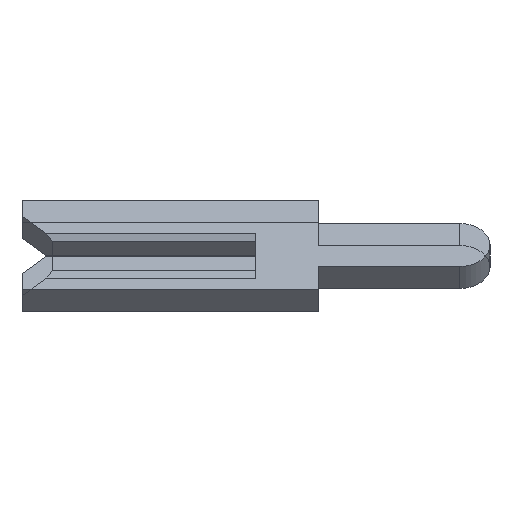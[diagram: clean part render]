
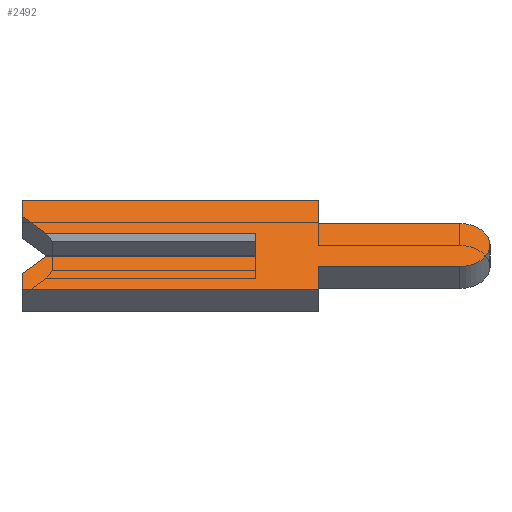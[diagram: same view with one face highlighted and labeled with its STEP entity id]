
A CAD part, left-side view. The second image highlights one B-rep face of the part: STEP entity #2492.
In plain terms, the highlighted face is planar.
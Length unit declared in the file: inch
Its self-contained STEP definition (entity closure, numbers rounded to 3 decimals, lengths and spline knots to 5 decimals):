
#36 = CARTESIAN_POINT ( 'NONE',  ( -0.01, 0.15, -0.04 ) ) ;
#107 = EDGE_CURVE ( 'NONE', #3180, #2590, #1143, .T. ) ;
#114 = CARTESIAN_POINT ( 'NONE',  ( -0.01, -0.04, 0.04 ) ) ;
#148 = VECTOR ( 'NONE', #1186, 39.37008 ) ;
#223 = ORIENTED_EDGE ( 'NONE', *, *, #336, .F. ) ;
#240 = ORIENTED_EDGE ( 'NONE', *, *, #3770, .F. ) ;
#252 = CARTESIAN_POINT ( 'NONE',  ( -0.01, 0.134, 0.01 ) ) ;
#256 = LINE ( 'NONE', #728, #2222 ) ;
#263 = VERTEX_POINT ( 'NONE', #923 ) ;
#294 = CARTESIAN_POINT ( 'NONE',  ( -0.01, -0.1305, 0.0195 ) ) ;
#305 = VECTOR ( 'NONE', #3773, 39.37008 ) ;
#336 = EDGE_CURVE ( 'NONE', #2750, #3180, #2020, .T. ) ;
#363 = DIRECTION ( 'NONE',  ( 0., -1., 0. ) ) ;
#417 = LINE ( 'NONE', #1323, #3799 ) ;
#418 = CARTESIAN_POINT ( 'NONE',  ( -0.01, 0., -0.01 ) ) ;
#441 = LINE ( 'NONE', #848, #148 ) ;
#448 = CARTESIAN_POINT ( 'NONE',  ( -0.01, -0.04, -0.0195 ) ) ;
#514 = CARTESIAN_POINT ( 'NONE',  ( -0.01, 0.15, -0.026 ) ) ;
#549 = LINE ( 'NONE', #2681, #627 ) ;
#596 = CARTESIAN_POINT ( 'NONE',  ( -0.01, -0.1305, 0. ) ) ;
#627 = VECTOR ( 'NONE', #901, 39.37008 ) ;
#654 = DIRECTION ( 'NONE',  ( 0., 1., 0. ) ) ;
#665 = LINE ( 'NONE', #2844, #951 ) ;
#690 = EDGE_CURVE ( 'NONE', #2633, #2304, #3844, .T. ) ;
#728 = CARTESIAN_POINT ( 'NONE',  ( -0.01, 0.15, 0.04 ) ) ;
#785 = CARTESIAN_POINT ( 'NONE',  ( -0.01, 0.15, -0.04 ) ) ;
#789 = ORIENTED_EDGE ( 'NONE', *, *, #107, .F. ) ;
#848 = CARTESIAN_POINT ( 'NONE',  ( -0.01, -0.04, -0.0195 ) ) ;
#854 = CIRCLE ( 'NONE', #2845, 0.0195 ) ;
#872 = EDGE_CURVE ( 'NONE', #2750, #1251, #417, .T. ) ;
#901 = DIRECTION ( 'NONE',  ( 0., -1., 0. ) ) ;
#919 = CARTESIAN_POINT ( 'NONE',  ( -0.01, 0.15, 0.026 ) ) ;
#923 = CARTESIAN_POINT ( 'NONE',  ( -0.01, -0.1305, -0.0195 ) ) ;
#929 = DIRECTION ( 'NONE',  ( 1., 0., 0. ) ) ;
#931 = VECTOR ( 'NONE', #654, 39.37008 ) ;
#951 = VECTOR ( 'NONE', #2807, 39.37008 ) ;
#999 = EDGE_CURVE ( 'NONE', #2590, #2348, #256, .T. ) ;
#1027 = EDGE_CURVE ( 'NONE', #2304, #2015, #2981, .T. ) ;
#1065 = ORIENTED_EDGE ( 'NONE', *, *, #1729, .F. ) ;
#1084 = CARTESIAN_POINT ( 'NONE',  ( -0.01, -0.04, -0.04 ) ) ;
#1143 = LINE ( 'NONE', #2137, #2611 ) ;
#1186 = DIRECTION ( 'NONE',  ( 0., 1., 0. ) ) ;
#1193 = ORIENTED_EDGE ( 'NONE', *, *, #2713, .F. ) ;
#1248 = DIRECTION ( 'NONE',  ( 0., 0.707, 0.707 ) ) ;
#1251 = VERTEX_POINT ( 'NONE', #2852 ) ;
#1310 = VECTOR ( 'NONE', #3634, 39.37008 ) ;
#1323 = CARTESIAN_POINT ( 'NONE',  ( -0.01, 0.15, 0.01 ) ) ;
#1350 = ORIENTED_EDGE ( 'NONE', *, *, #1027, .F. ) ;
#1370 = CARTESIAN_POINT ( 'NONE',  ( -0.01, 0.1305, -0.0065 ) ) ;
#1396 = VERTEX_POINT ( 'NONE', #448 ) ;
#1451 = EDGE_CURVE ( 'NONE', #1396, #2633, #3030, .T. ) ;
#1494 = CARTESIAN_POINT ( 'NONE',  ( -0.01, 0., 0.0065 ) ) ;
#1647 = EDGE_LOOP ( 'NONE', ( #1805, #1193, #2458, #1065, #1350, #3405, #2413, #3379, #3302, #240, #2543, #2516, #789, #223 ) ) ;
#1671 = CARTESIAN_POINT ( 'NONE',  ( -0.01, 0.15, -0.026 ) ) ;
#1729 = EDGE_CURVE ( 'NONE', #2015, #2900, #3544, .T. ) ;
#1781 = CARTESIAN_POINT ( 'NONE',  ( -0.01, -0.04, -0.04 ) ) ;
#1796 = DIRECTION ( 'NONE',  ( 1., 0., 0. ) ) ;
#1805 = ORIENTED_EDGE ( 'NONE', *, *, #872, .T. ) ;
#1866 = CARTESIAN_POINT ( 'NONE',  ( -0.01, -0.1305, 0. ) ) ;
#2015 = VERTEX_POINT ( 'NONE', #514 ) ;
#2020 = LINE ( 'NONE', #3032, #3547 ) ;
#2052 = PLANE ( 'NONE',  #3288 ) ;
#2083 = DIRECTION ( 'NONE',  ( 0., 0., -1. ) ) ;
#2137 = CARTESIAN_POINT ( 'NONE',  ( -0.01, 0.15, 0.026 ) ) ;
#2222 = VECTOR ( 'NONE', #3177, 39.37008 ) ;
#2225 = VECTOR ( 'NONE', #2865, 39.37008 ) ;
#2304 = VERTEX_POINT ( 'NONE', #785 ) ;
#2335 = CARTESIAN_POINT ( 'NONE',  ( -0.01, -0.04, 0.04 ) ) ;
#2348 = VERTEX_POINT ( 'NONE', #2335 ) ;
#2396 = LINE ( 'NONE', #1494, #1310 ) ;
#2413 = ORIENTED_EDGE ( 'NONE', *, *, #1451, .F. ) ;
#2442 = VERTEX_POINT ( 'NONE', #294 ) ;
#2458 = ORIENTED_EDGE ( 'NONE', *, *, #2512, .F. ) ;
#2467 = DIRECTION ( 'NONE',  ( 0., 0., 1. ) ) ;
#2492 = ADVANCED_FACE ( 'NONE', ( #3735 ), #2052, .F. ) ;
#2506 = DIRECTION ( 'NONE',  ( 0., 0., -1. ) ) ;
#2512 = EDGE_CURVE ( 'NONE', #2900, #3431, #549, .T. ) ;
#2516 = ORIENTED_EDGE ( 'NONE', *, *, #999, .F. ) ;
#2543 = ORIENTED_EDGE ( 'NONE', *, *, #3517, .F. ) ;
#2590 = VERTEX_POINT ( 'NONE', #3339 ) ;
#2611 = VECTOR ( 'NONE', #2467, 39.37008 ) ;
#2633 = VERTEX_POINT ( 'NONE', #1781 ) ;
#2681 = CARTESIAN_POINT ( 'NONE',  ( -0.01, -0.1305, -0.01 ) ) ;
#2713 = EDGE_CURVE ( 'NONE', #3431, #1251, #2396, .T. ) ;
#2717 = CARTESIAN_POINT ( 'NONE',  ( -0.01, -0.04, 0.0195 ) ) ;
#2719 = VECTOR ( 'NONE', #3262, 39.37008 ) ;
#2739 = EDGE_CURVE ( 'NONE', #263, #1396, #441, .T. ) ;
#2750 = VERTEX_POINT ( 'NONE', #252 ) ;
#2807 = DIRECTION ( 'NONE',  ( 0., -1., 0. ) ) ;
#2844 = CARTESIAN_POINT ( 'NONE',  ( -0.01, -0.04, 0.0195 ) ) ;
#2845 = AXIS2_PLACEMENT_3D ( 'NONE', #1866, #929, #3414 ) ;
#2852 = CARTESIAN_POINT ( 'NONE',  ( -0.01, 0., 0.01 ) ) ;
#2865 = DIRECTION ( 'NONE',  ( 0., 0., -1. ) ) ;
#2866 = VERTEX_POINT ( 'NONE', #2717 ) ;
#2900 = VERTEX_POINT ( 'NONE', #3074 ) ;
#2981 = LINE ( 'NONE', #1671, #305 ) ;
#3030 = LINE ( 'NONE', #1084, #2225 ) ;
#3032 = CARTESIAN_POINT ( 'NONE',  ( -0.01, 0.1305, 0.0065 ) ) ;
#3074 = CARTESIAN_POINT ( 'NONE',  ( -0.01, 0.134, -0.01 ) ) ;
#3096 = EDGE_CURVE ( 'NONE', #2442, #263, #854, .T. ) ;
#3177 = DIRECTION ( 'NONE',  ( 0., -1., 0. ) ) ;
#3180 = VERTEX_POINT ( 'NONE', #919 ) ;
#3262 = DIRECTION ( 'NONE',  ( 0., -0.707, 0.707 ) ) ;
#3288 = AXIS2_PLACEMENT_3D ( 'NONE', #596, #1796, #2083 ) ;
#3302 = ORIENTED_EDGE ( 'NONE', *, *, #3096, .F. ) ;
#3339 = CARTESIAN_POINT ( 'NONE',  ( -0.01, 0.15, 0.04 ) ) ;
#3379 = ORIENTED_EDGE ( 'NONE', *, *, #2739, .F. ) ;
#3405 = ORIENTED_EDGE ( 'NONE', *, *, #690, .F. ) ;
#3414 = DIRECTION ( 'NONE',  ( 0., 0., -1. ) ) ;
#3431 = VERTEX_POINT ( 'NONE', #418 ) ;
#3498 = VECTOR ( 'NONE', #2506, 39.37008 ) ;
#3517 = EDGE_CURVE ( 'NONE', #2348, #2866, #3782, .T. ) ;
#3544 = LINE ( 'NONE', #1370, #2719 ) ;
#3547 = VECTOR ( 'NONE', #1248, 39.37008 ) ;
#3634 = DIRECTION ( 'NONE',  ( 0., 0., 1. ) ) ;
#3735 = FACE_OUTER_BOUND ( 'NONE', #1647, .T. ) ;
#3770 = EDGE_CURVE ( 'NONE', #2866, #2442, #665, .T. ) ;
#3773 = DIRECTION ( 'NONE',  ( 0., 0., 1. ) ) ;
#3782 = LINE ( 'NONE', #114, #3498 ) ;
#3799 = VECTOR ( 'NONE', #363, 39.37008 ) ;
#3844 = LINE ( 'NONE', #36, #931 ) ;
